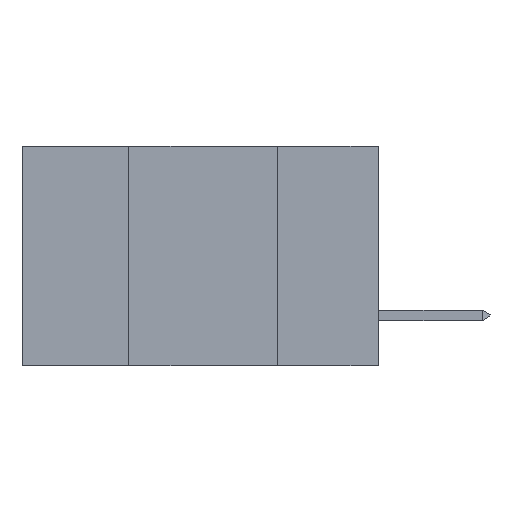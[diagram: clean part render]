
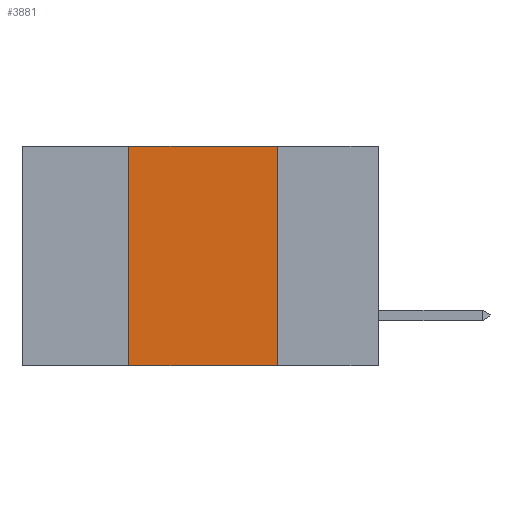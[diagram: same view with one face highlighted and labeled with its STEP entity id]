
A CAD part, left-side view. The second image highlights one B-rep face of the part: STEP entity #3881.
In plain terms, the highlighted planar face has unit normal (-1, 0, 0).
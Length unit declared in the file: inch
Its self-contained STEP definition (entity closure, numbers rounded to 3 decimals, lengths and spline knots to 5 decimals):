
#484 = CARTESIAN_POINT ( 'NONE',  ( 0., 0.6, 0. ) ) ;
#670 = DIRECTION ( 'NONE',  ( 0., 0., -1. ) ) ;
#795 = EDGE_CURVE ( 'NONE', #10413, #4776, #5063, .T. ) ;
#801 = EDGE_LOOP ( 'NONE', ( #7013, #1336, #5508, #7136 ) ) ;
#960 = VECTOR ( 'NONE', #10111, 39.37008 ) ;
#1336 = ORIENTED_EDGE ( 'NONE', *, *, #6606, .F. ) ;
#1417 = VECTOR ( 'NONE', #3373, 39.37008 ) ;
#1494 = CARTESIAN_POINT ( 'NONE',  ( 0., 0.17, -0.37 ) ) ;
#2489 = LINE ( 'NONE', #2648, #1417 ) ;
#2648 = CARTESIAN_POINT ( 'NONE',  ( 0., 0.42, -0.37 ) ) ;
#2677 = VERTEX_POINT ( 'NONE', #9014 ) ;
#2679 = LINE ( 'NONE', #8587, #960 ) ;
#3069 = DIRECTION ( 'NONE',  ( 0., 0., -1. ) ) ;
#3171 = EDGE_CURVE ( 'NONE', #10413, #2677, #2489, .T. ) ;
#3298 = LINE ( 'NONE', #1494, #10448 ) ;
#3373 = DIRECTION ( 'NONE',  ( 0., 0., 1. ) ) ;
#3881 = ADVANCED_FACE ( 'NONE', ( #8816 ), #4819, .F. ) ;
#4776 = VERTEX_POINT ( 'NONE', #5645 ) ;
#4819 = PLANE ( 'NONE',  #7002 ) ;
#4847 = EDGE_CURVE ( 'NONE', #8856, #4776, #3298, .T. ) ;
#5063 = LINE ( 'NONE', #9225, #5980 ) ;
#5120 = DIRECTION ( 'NONE',  ( 0., -1., 0. ) ) ;
#5508 = ORIENTED_EDGE ( 'NONE', *, *, #3171, .F. ) ;
#5645 = CARTESIAN_POINT ( 'NONE',  ( 0., 0.17, -0.37 ) ) ;
#5980 = VECTOR ( 'NONE', #5120, 39.37008 ) ;
#6606 = EDGE_CURVE ( 'NONE', #2677, #8856, #2679, .T. ) ;
#7002 = AXIS2_PLACEMENT_3D ( 'NONE', #484, #9573, #3069 ) ;
#7013 = ORIENTED_EDGE ( 'NONE', *, *, #4847, .F. ) ;
#7074 = CARTESIAN_POINT ( 'NONE',  ( 0., 0.17, 0. ) ) ;
#7136 = ORIENTED_EDGE ( 'NONE', *, *, #795, .T. ) ;
#7649 = CARTESIAN_POINT ( 'NONE',  ( 0., 0.42, -0.37 ) ) ;
#8587 = CARTESIAN_POINT ( 'NONE',  ( 0., 0.6, 0. ) ) ;
#8816 = FACE_OUTER_BOUND ( 'NONE', #801, .T. ) ;
#8856 = VERTEX_POINT ( 'NONE', #7074 ) ;
#9014 = CARTESIAN_POINT ( 'NONE',  ( 0., 0.42, 0. ) ) ;
#9225 = CARTESIAN_POINT ( 'NONE',  ( 0., 0.6, -0.37 ) ) ;
#9573 = DIRECTION ( 'NONE',  ( 1., 0., 0. ) ) ;
#10111 = DIRECTION ( 'NONE',  ( 0., -1., 0. ) ) ;
#10413 = VERTEX_POINT ( 'NONE', #7649 ) ;
#10448 = VECTOR ( 'NONE', #670, 39.37008 ) ;
